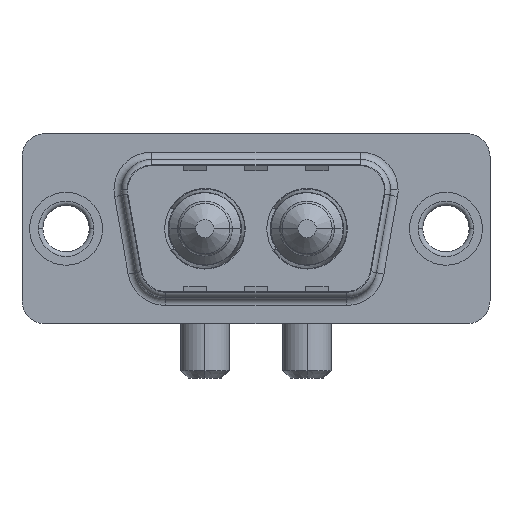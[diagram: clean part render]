
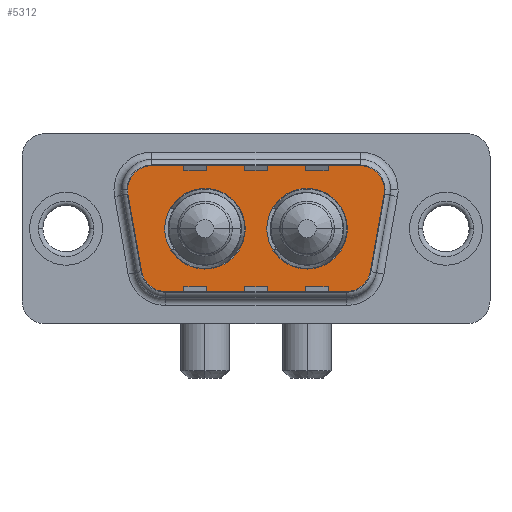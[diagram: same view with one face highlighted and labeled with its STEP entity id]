
A CAD part, top view. The second image highlights one B-rep face of the part: STEP entity #5312.
In plain terms, the highlighted planar face has unit normal (0, 0, 1).
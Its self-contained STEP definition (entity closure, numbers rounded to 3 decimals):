
#29 = CIRCLE ( 'NONE', #7145, 2. ) ;
#153 = FACE_BOUND ( 'NONE', #9264, .T. ) ;
#221 = VERTEX_POINT ( 'NONE', #2249 ) ;
#232 = VERTEX_POINT ( 'NONE', #7696 ) ;
#265 = CARTESIAN_POINT ( 'NONE',  ( 21.534, 2.553, 0. ) ) ;
#351 = ORIENTED_EDGE ( 'NONE', *, *, #7282, .T. ) ;
#415 = DIRECTION ( 'NONE',  ( 0.174, -0.985, 0. ) ) ;
#557 = EDGE_CURVE ( 'NONE', #232, #4149, #9291, .T. ) ;
#560 = DIRECTION ( 'NONE',  ( -1., 0., 0. ) ) ;
#714 = CARTESIAN_POINT ( 'NONE',  ( 18.541, -4.9, 0. ) ) ;
#745 = CARTESIAN_POINT ( 'NONE',  ( 19.564, 2.9, 0. ) ) ;
#788 = DIRECTION ( 'NONE',  ( 0., 0., 1. ) ) ;
#865 = EDGE_LOOP ( 'NONE', ( #8035, #3779 ) ) ;
#1070 = CARTESIAN_POINT ( 'NONE',  ( 18.541, -2.9, 0. ) ) ;
#1126 = CIRCLE ( 'NONE', #5836, 2. ) ;
#1259 = AXIS2_PLACEMENT_3D ( 'NONE', #3069, #7672, #8496 ) ;
#1423 = DIRECTION ( 'NONE',  ( 0.174, 0.985, 0. ) ) ;
#1574 = CIRCLE ( 'NONE', #8059, 2.65 ) ;
#1644 = FACE_OUTER_BOUND ( 'NONE', #7894, .T. ) ;
#1740 = LINE ( 'NONE', #5647, #1899 ) ;
#1758 = AXIS2_PLACEMENT_3D ( 'NONE', #2870, #2177, #4404 ) ;
#1890 = CARTESIAN_POINT ( 'NONE',  ( 9.14, 0., 0. ) ) ;
#1899 = VECTOR ( 'NONE', #415, 1000. ) ;
#2003 = EDGE_CURVE ( 'NONE', #3353, #7484, #7586, .T. ) ;
#2012 = EDGE_CURVE ( 'NONE', #4149, #232, #9459, .T. ) ;
#2018 = CARTESIAN_POINT ( 'NONE',  ( 5.436, 4.9, 0. ) ) ;
#2053 = VERTEX_POINT ( 'NONE', #2086 ) ;
#2086 = CARTESIAN_POINT ( 'NONE',  ( 6.49, 0., 0. ) ) ;
#2150 = VERTEX_POINT ( 'NONE', #9730 ) ;
#2177 = DIRECTION ( 'NONE',  ( 0., 0., 1. ) ) ;
#2218 = EDGE_CURVE ( 'NONE', #7484, #221, #1740, .T. ) ;
#2249 = CARTESIAN_POINT ( 'NONE',  ( 4.489, -3.247, 0. ) ) ;
#2304 = CARTESIAN_POINT ( 'NONE',  ( 13.21, 0., 0. ) ) ;
#2418 = ORIENTED_EDGE ( 'NONE', *, *, #2540, .T. ) ;
#2540 = EDGE_CURVE ( 'NONE', #8014, #9470, #1126, .T. ) ;
#2608 = EDGE_CURVE ( 'NONE', #2053, #2150, #1574, .T. ) ;
#2768 = DIRECTION ( 'NONE',  ( 0., 0., 1. ) ) ;
#2870 = CARTESIAN_POINT ( 'NONE',  ( 5.436, 2.9, 0. ) ) ;
#2919 = AXIS2_PLACEMENT_3D ( 'NONE', #1890, #4752, #6177 ) ;
#2948 = CARTESIAN_POINT ( 'NONE',  ( 18.541, -2.9, 0. ) ) ;
#2951 = DIRECTION ( 'NONE',  ( 0., 0., 1. ) ) ;
#3043 = CARTESIAN_POINT ( 'NONE',  ( 6.459, -4.9, 0. ) ) ;
#3060 = CARTESIAN_POINT ( 'NONE',  ( 20.511, -3.247, 0. ) ) ;
#3069 = CARTESIAN_POINT ( 'NONE',  ( 15.86, 0., 0. ) ) ;
#3122 = DIRECTION ( 'NONE',  ( 0., 0., 1. ) ) ;
#3123 = FACE_BOUND ( 'NONE', #865, .T. ) ;
#3323 = DIRECTION ( 'NONE',  ( 1., 0., 0. ) ) ;
#3353 = VERTEX_POINT ( 'NONE', #9385 ) ;
#3447 = CARTESIAN_POINT ( 'NONE',  ( 19.564, 4.9, 0. ) ) ;
#3779 = ORIENTED_EDGE ( 'NONE', *, *, #2608, .F. ) ;
#3791 = VERTEX_POINT ( 'NONE', #714 ) ;
#3837 = DIRECTION ( 'NONE',  ( 1., 0., 0. ) ) ;
#3848 = AXIS2_PLACEMENT_3D ( 'NONE', #1070, #6872, #3323 ) ;
#3881 = VERTEX_POINT ( 'NONE', #265 ) ;
#3889 = EDGE_CURVE ( 'NONE', #3881, #8014, #29, .T. ) ;
#3902 = DIRECTION ( 'NONE',  ( -1., 0., 0. ) ) ;
#4149 = VERTEX_POINT ( 'NONE', #2304 ) ;
#4216 = CARTESIAN_POINT ( 'NONE',  ( 6.459, -2.9, 0. ) ) ;
#4218 = EDGE_CURVE ( 'NONE', #5908, #3791, #7541, .T. ) ;
#4314 = ORIENTED_EDGE ( 'NONE', *, *, #2012, .F. ) ;
#4404 = DIRECTION ( 'NONE',  ( 1., 0., 0. ) ) ;
#4539 = CARTESIAN_POINT ( 'NONE',  ( 9.14, 0., 0. ) ) ;
#4579 = CARTESIAN_POINT ( 'NONE',  ( 21.534, 2.553, 0. ) ) ;
#4607 = CIRCLE ( 'NONE', #5554, 2. ) ;
#4752 = DIRECTION ( 'NONE',  ( 0., 0., 1. ) ) ;
#4771 = ORIENTED_EDGE ( 'NONE', *, *, #557, .F. ) ;
#4887 = DIRECTION ( 'NONE',  ( -1., 0., 0. ) ) ;
#5141 = ORIENTED_EDGE ( 'NONE', *, *, #2218, .T. ) ;
#5228 = DIRECTION ( 'NONE',  ( 0., 0., 1. ) ) ;
#5310 = ORIENTED_EDGE ( 'NONE', *, *, #4218, .T. ) ;
#5312 = ADVANCED_FACE ( 'NONE', ( #153, #3123, #1644 ), #8555, .T. ) ;
#5398 = VECTOR ( 'NONE', #3837, 1000. ) ;
#5554 = AXIS2_PLACEMENT_3D ( 'NONE', #4216, #2768, #560 ) ;
#5647 = CARTESIAN_POINT ( 'NONE',  ( 3.466, 2.553, 0. ) ) ;
#5658 = ORIENTED_EDGE ( 'NONE', *, *, #9111, .T. ) ;
#5836 = AXIS2_PLACEMENT_3D ( 'NONE', #745, #788, #3902 ) ;
#5908 = VERTEX_POINT ( 'NONE', #7230 ) ;
#5967 = DIRECTION ( 'NONE',  ( 1., 0., 0. ) ) ;
#6092 = EDGE_CURVE ( 'NONE', #3791, #7429, #9405, .T. ) ;
#6177 = DIRECTION ( 'NONE',  ( 1., 0., 0. ) ) ;
#6266 = CARTESIAN_POINT ( 'NONE',  ( 3.466, 2.553, 0. ) ) ;
#6356 = DIRECTION ( 'NONE',  ( 0., 0., 1. ) ) ;
#6531 = VECTOR ( 'NONE', #1423, 1000. ) ;
#6662 = ORIENTED_EDGE ( 'NONE', *, *, #6092, .T. ) ;
#6665 = VECTOR ( 'NONE', #4887, 1000. ) ;
#6710 = LINE ( 'NONE', #4579, #6531 ) ;
#6791 = AXIS2_PLACEMENT_3D ( 'NONE', #8941, #6356, #8211 ) ;
#6800 = ORIENTED_EDGE ( 'NONE', *, *, #3889, .T. ) ;
#6872 = DIRECTION ( 'NONE',  ( 0., 0., 1. ) ) ;
#7037 = EDGE_CURVE ( 'NONE', #2150, #2053, #9065, .T. ) ;
#7145 = AXIS2_PLACEMENT_3D ( 'NONE', #9196, #3122, #9089 ) ;
#7230 = CARTESIAN_POINT ( 'NONE',  ( 6.459, -4.9, 0. ) ) ;
#7282 = EDGE_CURVE ( 'NONE', #221, #5908, #4607, .T. ) ;
#7319 = LINE ( 'NONE', #2018, #6665 ) ;
#7429 = VERTEX_POINT ( 'NONE', #3060 ) ;
#7484 = VERTEX_POINT ( 'NONE', #6266 ) ;
#7541 = LINE ( 'NONE', #3043, #5398 ) ;
#7586 = CIRCLE ( 'NONE', #1758, 2. ) ;
#7672 = DIRECTION ( 'NONE',  ( 0., 0., 1. ) ) ;
#7696 = CARTESIAN_POINT ( 'NONE',  ( 18.51, 0., 0. ) ) ;
#7697 = EDGE_CURVE ( 'NONE', #9470, #3353, #7319, .T. ) ;
#7701 = CARTESIAN_POINT ( 'NONE',  ( 21.564, 2.9, 0. ) ) ;
#7894 = EDGE_LOOP ( 'NONE', ( #6662, #5658, #6800, #2418, #8903, #8708, #5141, #351, #5310 ) ) ;
#8014 = VERTEX_POINT ( 'NONE', #7701 ) ;
#8035 = ORIENTED_EDGE ( 'NONE', *, *, #7037, .F. ) ;
#8059 = AXIS2_PLACEMENT_3D ( 'NONE', #4539, #2951, #5967 ) ;
#8211 = DIRECTION ( 'NONE',  ( 1., 0., 0. ) ) ;
#8249 = DIRECTION ( 'NONE',  ( 1., 0., 0. ) ) ;
#8496 = DIRECTION ( 'NONE',  ( 1., 0., 0. ) ) ;
#8555 = PLANE ( 'NONE',  #3848 ) ;
#8708 = ORIENTED_EDGE ( 'NONE', *, *, #2003, .T. ) ;
#8763 = AXIS2_PLACEMENT_3D ( 'NONE', #2948, #5228, #8249 ) ;
#8903 = ORIENTED_EDGE ( 'NONE', *, *, #7697, .T. ) ;
#8941 = CARTESIAN_POINT ( 'NONE',  ( 15.86, 0., 0. ) ) ;
#9065 = CIRCLE ( 'NONE', #2919, 2.65 ) ;
#9089 = DIRECTION ( 'NONE',  ( -1., 0., 0. ) ) ;
#9111 = EDGE_CURVE ( 'NONE', #7429, #3881, #6710, .T. ) ;
#9196 = CARTESIAN_POINT ( 'NONE',  ( 19.564, 2.9, 0. ) ) ;
#9264 = EDGE_LOOP ( 'NONE', ( #4771, #4314 ) ) ;
#9291 = CIRCLE ( 'NONE', #1259, 2.65 ) ;
#9385 = CARTESIAN_POINT ( 'NONE',  ( 5.436, 4.9, 0. ) ) ;
#9405 = CIRCLE ( 'NONE', #8763, 2. ) ;
#9459 = CIRCLE ( 'NONE', #6791, 2.65 ) ;
#9470 = VERTEX_POINT ( 'NONE', #3447 ) ;
#9730 = CARTESIAN_POINT ( 'NONE',  ( 11.79, 0., 0. ) ) ;
